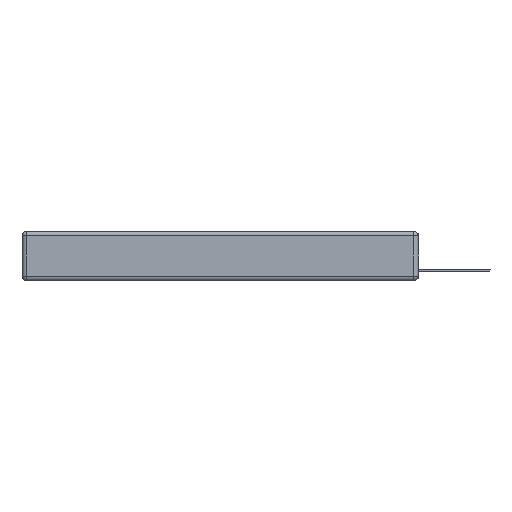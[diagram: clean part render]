
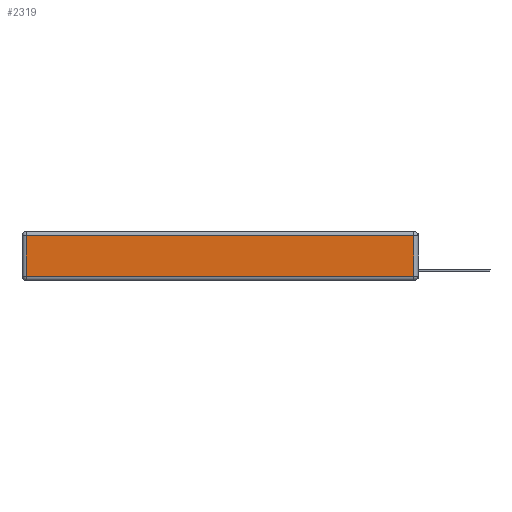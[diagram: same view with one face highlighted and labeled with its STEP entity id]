
A CAD part, left-side view. The second image highlights one B-rep face of the part: STEP entity #2319.
In plain terms, the highlighted planar face has unit normal (-1, 0, 0).
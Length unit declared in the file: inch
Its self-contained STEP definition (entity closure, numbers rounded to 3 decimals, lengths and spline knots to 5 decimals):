
#663 = VERTEX_POINT ( 'NONE', #11951 ) ;
#1131 = FACE_OUTER_BOUND ( 'NONE', #20699, .T. ) ;
#2020 = CARTESIAN_POINT ( 'NONE',  ( 0., 2.72, -0.313 ) ) ;
#2319 = ADVANCED_FACE ( 'NONE', ( #1131 ), #3064, .T. ) ;
#3064 = PLANE ( 'NONE',  #24088 ) ;
#3097 = CARTESIAN_POINT ( 'NONE',  ( 0., 0., -0.313 ) ) ;
#3898 = VERTEX_POINT ( 'NONE', #17386 ) ;
#4843 = VECTOR ( 'NONE', #15507, 39.37008 ) ;
#5011 = LINE ( 'NONE', #3097, #15986 ) ;
#6772 = ORIENTED_EDGE ( 'NONE', *, *, #25836, .T. ) ;
#6796 = LINE ( 'NONE', #11028, #21481 ) ;
#7071 = DIRECTION ( 'NONE',  ( 0., 0., -1. ) ) ;
#7191 = CARTESIAN_POINT ( 'NONE',  ( 0., 0.03, -0.343 ) ) ;
#9119 = CARTESIAN_POINT ( 'NONE',  ( 0., 2.72, -0.343 ) ) ;
#9504 = DIRECTION ( 'NONE',  ( 0., -1., 0. ) ) ;
#9616 = EDGE_CURVE ( 'NONE', #15059, #20757, #5011, .T. ) ;
#11028 = CARTESIAN_POINT ( 'NONE',  ( 0., 2.75, -0.03 ) ) ;
#11376 = CARTESIAN_POINT ( 'NONE',  ( 0., 0., -0.343 ) ) ;
#11951 = CARTESIAN_POINT ( 'NONE',  ( 0., 0.03, -0.03 ) ) ;
#12650 = DIRECTION ( 'NONE',  ( 0., 1., 0. ) ) ;
#14989 = LINE ( 'NONE', #9119, #22636 ) ;
#15059 = VERTEX_POINT ( 'NONE', #2020 ) ;
#15182 = EDGE_CURVE ( 'NONE', #3898, #15059, #14989, .T. ) ;
#15507 = DIRECTION ( 'NONE',  ( 0., 0., 1. ) ) ;
#15986 = VECTOR ( 'NONE', #9504, 39.37008 ) ;
#17386 = CARTESIAN_POINT ( 'NONE',  ( 0., 2.72, -0.03 ) ) ;
#17653 = DIRECTION ( 'NONE',  ( -1., 0., 0. ) ) ;
#18546 = ORIENTED_EDGE ( 'NONE', *, *, #9616, .T. ) ;
#19522 = ORIENTED_EDGE ( 'NONE', *, *, #22624, .T. ) ;
#20699 = EDGE_LOOP ( 'NONE', ( #18546, #19522, #6772, #25122 ) ) ;
#20757 = VERTEX_POINT ( 'NONE', #26327 ) ;
#21481 = VECTOR ( 'NONE', #12650, 39.37008 ) ;
#22624 = EDGE_CURVE ( 'NONE', #20757, #663, #25894, .T. ) ;
#22636 = VECTOR ( 'NONE', #7071, 39.37008 ) ;
#24088 = AXIS2_PLACEMENT_3D ( 'NONE', #11376, #17653, #25991 ) ;
#25122 = ORIENTED_EDGE ( 'NONE', *, *, #15182, .T. ) ;
#25836 = EDGE_CURVE ( 'NONE', #663, #3898, #6796, .T. ) ;
#25894 = LINE ( 'NONE', #7191, #4843 ) ;
#25991 = DIRECTION ( 'NONE',  ( 0., 0., 1. ) ) ;
#26327 = CARTESIAN_POINT ( 'NONE',  ( 0., 0.03, -0.313 ) ) ;
